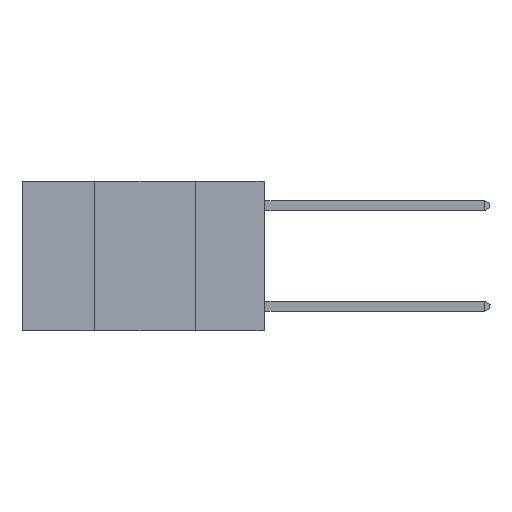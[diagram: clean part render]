
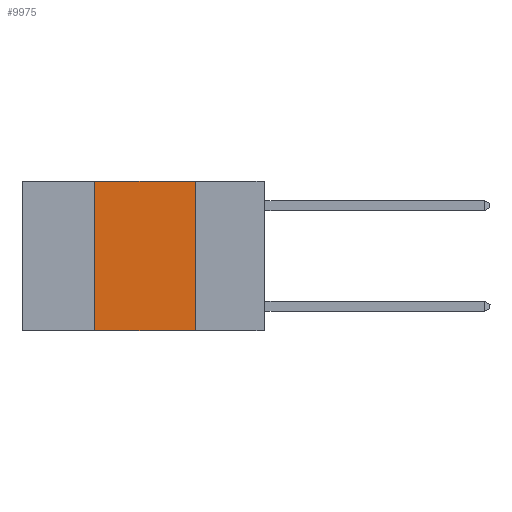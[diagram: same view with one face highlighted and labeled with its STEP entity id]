
A CAD part, left-side view. The second image highlights one B-rep face of the part: STEP entity #9975.
In plain terms, the highlighted planar face has unit normal (-1, 0, 0).
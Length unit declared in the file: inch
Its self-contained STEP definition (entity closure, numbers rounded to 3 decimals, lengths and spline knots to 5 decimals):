
#1090 = CARTESIAN_POINT ( 'NONE',  ( 0., 0.6, 0. ) ) ;
#1669 = CARTESIAN_POINT ( 'NONE',  ( 0., 0.6, -0.37 ) ) ;
#1904 = VERTEX_POINT ( 'NONE', #6486 ) ;
#2989 = LINE ( 'NONE', #23578, #23313 ) ;
#5505 = PLANE ( 'NONE',  #22000 ) ;
#5509 = VERTEX_POINT ( 'NONE', #25321 ) ;
#5539 = ORIENTED_EDGE ( 'NONE', *, *, #16490, .F. ) ;
#6079 = VECTOR ( 'NONE', #17076, 39.37008 ) ;
#6486 = CARTESIAN_POINT ( 'NONE',  ( 0., 0.17, -0.37 ) ) ;
#7333 = ORIENTED_EDGE ( 'NONE', *, *, #18309, .F. ) ;
#7508 = DIRECTION ( 'NONE',  ( 1., 0., 0. ) ) ;
#7535 = DIRECTION ( 'NONE',  ( 0., -1., 0. ) ) ;
#8026 = EDGE_LOOP ( 'NONE', ( #5539, #17692, #7333, #23039 ) ) ;
#8429 = VERTEX_POINT ( 'NONE', #14471 ) ;
#9975 = ADVANCED_FACE ( 'NONE', ( #19163 ), #5505, .F. ) ;
#11493 = VECTOR ( 'NONE', #19237, 39.37008 ) ;
#14471 = CARTESIAN_POINT ( 'NONE',  ( 0., 0.42, 0. ) ) ;
#16490 = EDGE_CURVE ( 'NONE', #22180, #1904, #2989, .T. ) ;
#17076 = DIRECTION ( 'NONE',  ( 0., -1., 0. ) ) ;
#17280 = CARTESIAN_POINT ( 'NONE',  ( 0., 0.42, 0. ) ) ;
#17692 = ORIENTED_EDGE ( 'NONE', *, *, #24481, .F. ) ;
#18309 = EDGE_CURVE ( 'NONE', #5509, #8429, #21976, .T. ) ;
#18910 = DIRECTION ( 'NONE',  ( 0., 0., -1. ) ) ;
#19163 = FACE_OUTER_BOUND ( 'NONE', #8026, .T. ) ;
#19237 = DIRECTION ( 'NONE',  ( 0., 0., 1. ) ) ;
#19290 = CARTESIAN_POINT ( 'NONE',  ( 0., 0.6, 0. ) ) ;
#21269 = DIRECTION ( 'NONE',  ( 0., 0., -1. ) ) ;
#21777 = LINE ( 'NONE', #1090, #6079 ) ;
#21976 = LINE ( 'NONE', #17280, #11493 ) ;
#22000 = AXIS2_PLACEMENT_3D ( 'NONE', #19290, #7508, #21269 ) ;
#22180 = VERTEX_POINT ( 'NONE', #24497 ) ;
#22431 = EDGE_CURVE ( 'NONE', #5509, #1904, #23446, .T. ) ;
#23039 = ORIENTED_EDGE ( 'NONE', *, *, #22431, .T. ) ;
#23313 = VECTOR ( 'NONE', #18910, 39.37008 ) ;
#23446 = LINE ( 'NONE', #1669, #24067 ) ;
#23578 = CARTESIAN_POINT ( 'NONE',  ( 0., 0.17, 0. ) ) ;
#24067 = VECTOR ( 'NONE', #7535, 39.37008 ) ;
#24481 = EDGE_CURVE ( 'NONE', #8429, #22180, #21777, .T. ) ;
#24497 = CARTESIAN_POINT ( 'NONE',  ( 0., 0.17, 0. ) ) ;
#25321 = CARTESIAN_POINT ( 'NONE',  ( 0., 0.42, -0.37 ) ) ;
